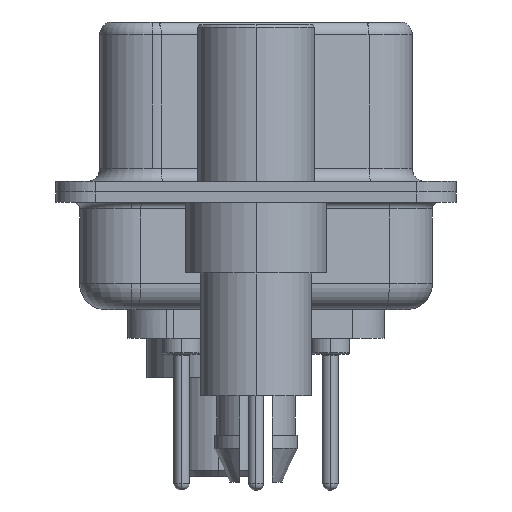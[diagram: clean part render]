
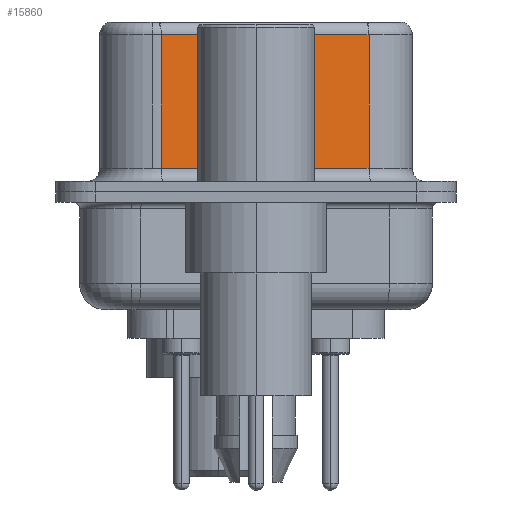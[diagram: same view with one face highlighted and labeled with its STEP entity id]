
A CAD part, left-side view. The second image highlights one B-rep face of the part: STEP entity #15860.
In plain terms, the highlighted planar face has unit normal (-0.985, -0.174, 0).
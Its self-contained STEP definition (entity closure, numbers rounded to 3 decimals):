
#528 = DIRECTION ( 'NONE',  ( 0.985, 0.174, 0. ) ) ;
#763 = CARTESIAN_POINT ( 'NONE',  ( 3.73, 3.628, 6.52 ) ) ;
#1332 = EDGE_CURVE ( 'NONE', #26103, #8345, #15573, .T. ) ;
#2464 = LINE ( 'NONE', #17869, #25468 ) ;
#2622 = VECTOR ( 'NONE', #31316, 1000. ) ;
#2922 = EDGE_CURVE ( 'NONE', #8345, #22136, #4836, .T. ) ;
#3006 = VECTOR ( 'NONE', #16199, 1000. ) ;
#4836 = LINE ( 'NONE', #13489, #10558 ) ;
#5615 = DIRECTION ( 'NONE',  ( 0.174, -0.985, 0. ) ) ;
#8345 = VERTEX_POINT ( 'NONE', #9812 ) ;
#9505 = LINE ( 'NONE', #18543, #3006 ) ;
#9812 = CARTESIAN_POINT ( 'NONE',  ( 3.73, 3.628, 0.9 ) ) ;
#10558 = VECTOR ( 'NONE', #5615, 1000. ) ;
#11152 = EDGE_LOOP ( 'NONE', ( #23407, #17567, #28340, #25005 ) ) ;
#11207 = AXIS2_PLACEMENT_3D ( 'NONE', #12667, #528, #17576 ) ;
#12667 = CARTESIAN_POINT ( 'NONE',  ( 5.132, -4.322, 6.52 ) ) ;
#13489 = CARTESIAN_POINT ( 'NONE',  ( 5.132, -4.322, 0.9 ) ) ;
#14104 = CARTESIAN_POINT ( 'NONE',  ( 5.132, -4.322, 0.9 ) ) ;
#15573 = LINE ( 'NONE', #763, #2622 ) ;
#15860 = ADVANCED_FACE ( 'NONE', ( #16388 ), #30012, .F. ) ;
#16199 = DIRECTION ( 'NONE',  ( -0.174, 0.985, 0. ) ) ;
#16388 = FACE_OUTER_BOUND ( 'NONE', #11152, .T. ) ;
#17567 = ORIENTED_EDGE ( 'NONE', *, *, #28344, .T. ) ;
#17576 = DIRECTION ( 'NONE',  ( -0.174, 0.985, 0. ) ) ;
#17869 = CARTESIAN_POINT ( 'NONE',  ( 5.132, -4.322, 6.52 ) ) ;
#17963 = CARTESIAN_POINT ( 'NONE',  ( 3.73, 3.628, 6.02 ) ) ;
#18543 = CARTESIAN_POINT ( 'NONE',  ( 5.132, -4.322, 6.02 ) ) ;
#22136 = VERTEX_POINT ( 'NONE', #14104 ) ;
#23407 = ORIENTED_EDGE ( 'NONE', *, *, #24267, .F. ) ;
#23740 = VERTEX_POINT ( 'NONE', #25559 ) ;
#24267 = EDGE_CURVE ( 'NONE', #23740, #22136, #2464, .T. ) ;
#25005 = ORIENTED_EDGE ( 'NONE', *, *, #2922, .T. ) ;
#25367 = DIRECTION ( 'NONE',  ( 0., 0., -1. ) ) ;
#25468 = VECTOR ( 'NONE', #25367, 1000. ) ;
#25559 = CARTESIAN_POINT ( 'NONE',  ( 5.132, -4.322, 6.02 ) ) ;
#26103 = VERTEX_POINT ( 'NONE', #17963 ) ;
#28340 = ORIENTED_EDGE ( 'NONE', *, *, #1332, .T. ) ;
#28344 = EDGE_CURVE ( 'NONE', #23740, #26103, #9505, .T. ) ;
#30012 = PLANE ( 'NONE',  #11207 ) ;
#31316 = DIRECTION ( 'NONE',  ( 0., 0., -1. ) ) ;
